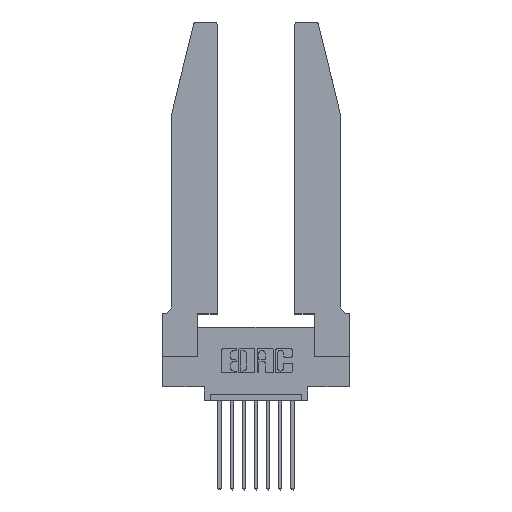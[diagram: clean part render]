
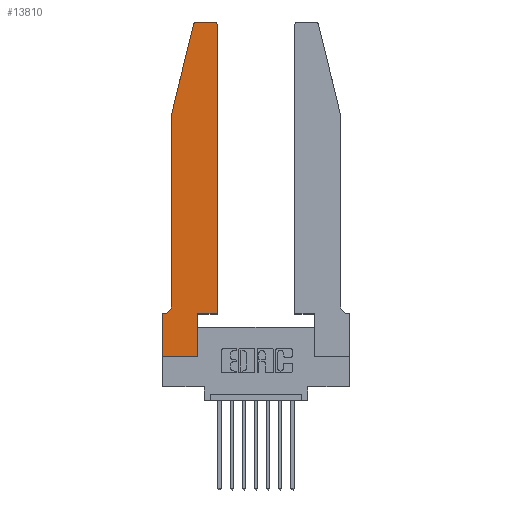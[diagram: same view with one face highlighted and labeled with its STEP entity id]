
A CAD part, top view. The second image highlights one B-rep face of the part: STEP entity #13810.
In plain terms, the highlighted planar face has unit normal (0, 0, 1).
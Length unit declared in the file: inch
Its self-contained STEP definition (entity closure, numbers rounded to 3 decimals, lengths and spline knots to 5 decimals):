
#51 = CARTESIAN_POINT ( 'NONE',  ( 0.0755, 2., 0.37 ) ) ;
#203 = VECTOR ( 'NONE', #13954, 39.37008 ) ;
#235 = EDGE_CURVE ( 'NONE', #3041, #14117, #14457, .T. ) ;
#490 = CARTESIAN_POINT ( 'NONE',  ( 0.4205, 2.72, 0.37 ) ) ;
#508 = VERTEX_POINT ( 'NONE', #7879 ) ;
#536 = DIRECTION ( 'NONE',  ( 0., 0., 1. ) ) ;
#558 = LINE ( 'NONE', #3462, #13480 ) ;
#617 = EDGE_CURVE ( 'NONE', #2372, #5224, #14794, .T. ) ;
#665 = EDGE_CURVE ( 'NONE', #913, #3041, #9237, .T. ) ;
#913 = VERTEX_POINT ( 'NONE', #12996 ) ;
#1173 = CARTESIAN_POINT ( 'NONE',  ( 0., 0., 0.37 ) ) ;
#1214 = ORIENTED_EDGE ( 'NONE', *, *, #12410, .T. ) ;
#1285 = CIRCLE ( 'NONE', #12989, 0.03 ) ;
#1289 = CARTESIAN_POINT ( 'NONE',  ( 0.0755, 2., 0.37 ) ) ;
#1714 = CARTESIAN_POINT ( 'NONE',  ( 0.4205, 2.75, 0.37 ) ) ;
#1715 = LINE ( 'NONE', #3823, #2426 ) ;
#1923 = EDGE_CURVE ( 'NONE', #6200, #508, #8995, .T. ) ;
#1992 = DIRECTION ( 'NONE',  ( 1., 0., 0. ) ) ;
#2226 = ORIENTED_EDGE ( 'NONE', *, *, #7973, .T. ) ;
#2351 = VECTOR ( 'NONE', #14024, 39.37008 ) ;
#2372 = VERTEX_POINT ( 'NONE', #14715 ) ;
#2426 = VECTOR ( 'NONE', #10908, 39.37008 ) ;
#2472 = VERTEX_POINT ( 'NONE', #3130 ) ;
#2528 = VERTEX_POINT ( 'NONE', #7537 ) ;
#2912 = FACE_OUTER_BOUND ( 'NONE', #11536, .T. ) ;
#3041 = VERTEX_POINT ( 'NONE', #14023 ) ;
#3071 = ORIENTED_EDGE ( 'NONE', *, *, #617, .T. ) ;
#3130 = CARTESIAN_POINT ( 'NONE',  ( 0.4505, 2.72, 0.37 ) ) ;
#3462 = CARTESIAN_POINT ( 'NONE',  ( 0.4505, 0.35, 0.37 ) ) ;
#3823 = CARTESIAN_POINT ( 'NONE',  ( 0., 0., 0.37 ) ) ;
#4121 = DIRECTION ( 'NONE',  ( 0., 0., 1. ) ) ;
#4279 = AXIS2_PLACEMENT_3D ( 'NONE', #6774, #10260, #6721 ) ;
#4325 = ORIENTED_EDGE ( 'NONE', *, *, #4991, .T. ) ;
#4850 = VERTEX_POINT ( 'NONE', #1714 ) ;
#4991 = EDGE_CURVE ( 'NONE', #6484, #6200, #12120, .T. ) ;
#5224 = VERTEX_POINT ( 'NONE', #10377 ) ;
#5307 = ORIENTED_EDGE ( 'NONE', *, *, #7986, .T. ) ;
#5427 = ORIENTED_EDGE ( 'NONE', *, *, #12052, .T. ) ;
#5678 = DIRECTION ( 'NONE',  ( 0., 1., 0. ) ) ;
#5766 = CARTESIAN_POINT ( 'NONE',  ( 0.284, 2.72, 0.37 ) ) ;
#5785 = DIRECTION ( 'NONE',  ( -1., 0., 0. ) ) ;
#6200 = VERTEX_POINT ( 'NONE', #12193 ) ;
#6227 = ORIENTED_EDGE ( 'NONE', *, *, #7487, .T. ) ;
#6376 = VECTOR ( 'NONE', #1992, 39.37008 ) ;
#6484 = VERTEX_POINT ( 'NONE', #1173 ) ;
#6721 = DIRECTION ( 'NONE',  ( -1., 0., 0. ) ) ;
#6774 = CARTESIAN_POINT ( 'NONE',  ( 0.0055, 0.42, 0.37 ) ) ;
#7202 = VECTOR ( 'NONE', #11609, 39.37008 ) ;
#7386 = ORIENTED_EDGE ( 'NONE', *, *, #1923, .T. ) ;
#7487 = EDGE_CURVE ( 'NONE', #2472, #4850, #1285, .T. ) ;
#7537 = CARTESIAN_POINT ( 'NONE',  ( 0.4505, 0.35, 0.37 ) ) ;
#7624 = LINE ( 'NONE', #1289, #2351 ) ;
#7667 = LINE ( 'NONE', #11599, #11778 ) ;
#7879 = CARTESIAN_POINT ( 'NONE',  ( 0.2865, 0.35, 0.37 ) ) ;
#7931 = VERTEX_POINT ( 'NONE', #9348 ) ;
#7973 = EDGE_CURVE ( 'NONE', #5224, #7931, #9700, .T. ) ;
#7986 = EDGE_CURVE ( 'NONE', #2528, #2472, #558, .T. ) ;
#8413 = DIRECTION ( 'NONE',  ( 1., 0., 0. ) ) ;
#8507 = DIRECTION ( 'NONE',  ( 1., 0., 0. ) ) ;
#8849 = CARTESIAN_POINT ( 'NONE',  ( 0.0755, 0.35, 0.37 ) ) ;
#8995 = LINE ( 'NONE', #12733, #203 ) ;
#9237 = CIRCLE ( 'NONE', #4279, 0.07 ) ;
#9348 = CARTESIAN_POINT ( 'NONE',  ( 0.0755, 2., 0.37 ) ) ;
#9636 = DIRECTION ( 'NONE',  ( 1., 0., 0. ) ) ;
#9700 = LINE ( 'NONE', #51, #7202 ) ;
#9771 = VECTOR ( 'NONE', #5785, 39.37008 ) ;
#10260 = DIRECTION ( 'NONE',  ( 0., 0., -1. ) ) ;
#10335 = ORIENTED_EDGE ( 'NONE', *, *, #235, .T. ) ;
#10346 = DIRECTION ( 'NONE',  ( -1., 0., 0. ) ) ;
#10377 = CARTESIAN_POINT ( 'NONE',  ( 0.25487, 2.72718, 0.37 ) ) ;
#10385 = ORIENTED_EDGE ( 'NONE', *, *, #665, .T. ) ;
#10405 = CARTESIAN_POINT ( 'NONE',  ( 0., 0.35, 0.37 ) ) ;
#10908 = DIRECTION ( 'NONE',  ( 0., -1., 0. ) ) ;
#11536 = EDGE_LOOP ( 'NONE', ( #1214, #3071, #2226, #12505, #10385, #10335, #5427, #4325, #7386, #14101, #5307, #6227 ) ) ;
#11579 = EDGE_CURVE ( 'NONE', #7931, #913, #7624, .T. ) ;
#11599 = CARTESIAN_POINT ( 'NONE',  ( 0.2605, 2.75, 0.37 ) ) ;
#11609 = DIRECTION ( 'NONE',  ( -0.239, -0.971, 0. ) ) ;
#11778 = VECTOR ( 'NONE', #10346, 39.37008 ) ;
#12009 = PLANE ( 'NONE',  #12655 ) ;
#12052 = EDGE_CURVE ( 'NONE', #14117, #6484, #1715, .T. ) ;
#12080 = EDGE_CURVE ( 'NONE', #508, #2528, #13916, .T. ) ;
#12120 = LINE ( 'NONE', #14685, #6376 ) ;
#12193 = CARTESIAN_POINT ( 'NONE',  ( 0.2865, 0., 0.37 ) ) ;
#12410 = EDGE_CURVE ( 'NONE', #4850, #2372, #7667, .T. ) ;
#12505 = ORIENTED_EDGE ( 'NONE', *, *, #11579, .T. ) ;
#12655 = AXIS2_PLACEMENT_3D ( 'NONE', #13253, #4121, #8507 ) ;
#12733 = CARTESIAN_POINT ( 'NONE',  ( 0.2865, 0.35, 0.37 ) ) ;
#12989 = AXIS2_PLACEMENT_3D ( 'NONE', #490, #536, #8413 ) ;
#12995 = CARTESIAN_POINT ( 'NONE',  ( 0.4505, 0.35, 0.37 ) ) ;
#12996 = CARTESIAN_POINT ( 'NONE',  ( 0.0755, 0.42, 0.37 ) ) ;
#13253 = CARTESIAN_POINT ( 'NONE',  ( 0., 0.35, 0.37 ) ) ;
#13480 = VECTOR ( 'NONE', #5678, 39.37008 ) ;
#13810 = ADVANCED_FACE ( 'NONE', ( #2912 ), #12009, .T. ) ;
#13916 = LINE ( 'NONE', #12995, #14291 ) ;
#13954 = DIRECTION ( 'NONE',  ( 0., 1., 0. ) ) ;
#14003 = AXIS2_PLACEMENT_3D ( 'NONE', #5766, #14343, #14649 ) ;
#14023 = CARTESIAN_POINT ( 'NONE',  ( 0.0055, 0.35, 0.37 ) ) ;
#14024 = DIRECTION ( 'NONE',  ( 0., -1., 0. ) ) ;
#14101 = ORIENTED_EDGE ( 'NONE', *, *, #12080, .T. ) ;
#14117 = VERTEX_POINT ( 'NONE', #10405 ) ;
#14291 = VECTOR ( 'NONE', #9636, 39.37008 ) ;
#14343 = DIRECTION ( 'NONE',  ( 0., 0., 1. ) ) ;
#14457 = LINE ( 'NONE', #8849, #9771 ) ;
#14649 = DIRECTION ( 'NONE',  ( 1., 0., 0. ) ) ;
#14685 = CARTESIAN_POINT ( 'NONE',  ( 0., 0., 0.37 ) ) ;
#14715 = CARTESIAN_POINT ( 'NONE',  ( 0.284, 2.75, 0.37 ) ) ;
#14794 = CIRCLE ( 'NONE', #14003, 0.03 ) ;
